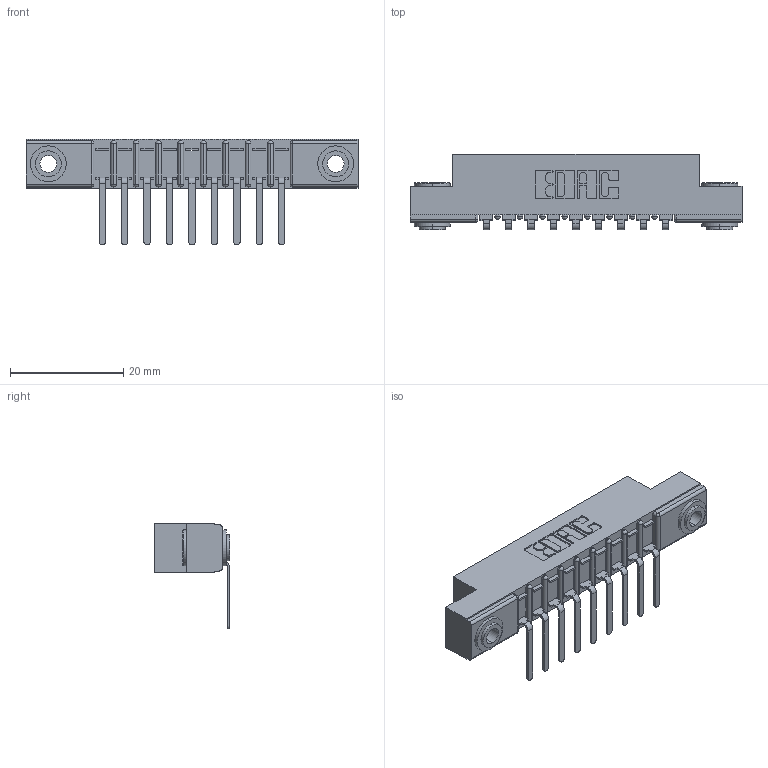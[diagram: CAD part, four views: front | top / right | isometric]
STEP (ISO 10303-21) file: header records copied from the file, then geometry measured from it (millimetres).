
FILE_DESCRIPTION (( 'STEP AP203' ), '1' );
FILE_NAME ('357-009-557-103.STEP', '2018-08-07T02:19:08', ( '' ), ( '' ), 'SwSTEP 2.0', 'SolidWorks 2016', '' );
FILE_SCHEMA (( 'CONFIG_CONTROL_DESIGN' ));
Length unit declared in the file: inch
Products named in the file (4): 307-290-002_557; 345-250-002_345-250-002-102; 357-009-557-103; 307 Part_.156 Dia Mounting Holes
Assembly tree (12 placements, depth 2):
  357-009-557-103
    307 Part_.156 Dia Mounting Holes
    307-290-002_557  x9
    345-250-002_345-250-002-102  x2
Bounding box: 58.67 x 13.36 x 18.67 mm (x, y, z)
Volume: 3892.3 mm3; surface area: 6749 mm2
Topology: 12 solids, 12 shells, 882 faces, 2631 edges, 1722 vertices
Faces by surface type: plane 517, cylinder 337, sphere 20, cone 8
Entity records: 13703 total; most frequent: CARTESIAN_POINT 2285, ORIENTED_EDGE 2266, DIRECTION 2251, EDGE_CURVE 1133, LINE 843, VECTOR 843, VERTEX_POINT 738, AXIS2_PLACEMENT_3D 704
